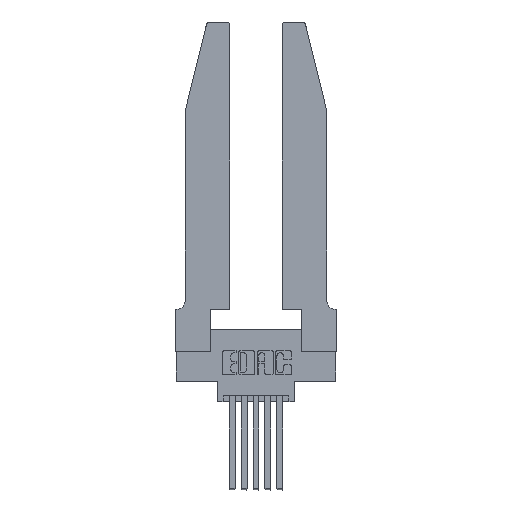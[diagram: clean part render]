
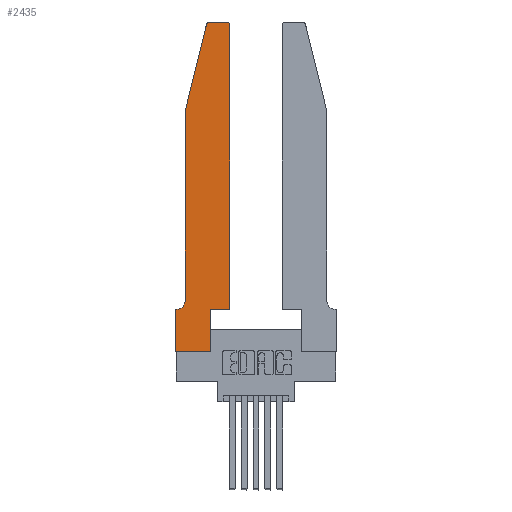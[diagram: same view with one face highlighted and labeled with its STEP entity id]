
A CAD part, top view. The second image highlights one B-rep face of the part: STEP entity #2435.
In plain terms, the highlighted planar face has unit normal (0, 0, 1).
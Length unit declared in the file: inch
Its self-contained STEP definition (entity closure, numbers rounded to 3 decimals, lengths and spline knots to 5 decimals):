
#417 = VERTEX_POINT ( 'NONE', #3624 ) ;
#426 = CARTESIAN_POINT ( 'NONE',  ( 0., 0., 0.37 ) ) ;
#519 = ORIENTED_EDGE ( 'NONE', *, *, #11851, .T. ) ;
#728 = VERTEX_POINT ( 'NONE', #12344 ) ;
#808 = EDGE_CURVE ( 'NONE', #11950, #12242, #9033, .T. ) ;
#812 = CARTESIAN_POINT ( 'NONE',  ( 0., 0., 0.37 ) ) ;
#825 = VECTOR ( 'NONE', #11538, 39.37008 ) ;
#841 = DIRECTION ( 'NONE',  ( 1., 0., 0. ) ) ;
#1068 = VERTEX_POINT ( 'NONE', #5139 ) ;
#1490 = CARTESIAN_POINT ( 'NONE',  ( 0.2605, 2.75, 0.37 ) ) ;
#1587 = ORIENTED_EDGE ( 'NONE', *, *, #10519, .T. ) ;
#1811 = DIRECTION ( 'NONE',  ( 0., -1., 0. ) ) ;
#1872 = VECTOR ( 'NONE', #1811, 39.37008 ) ;
#1958 = DIRECTION ( 'NONE',  ( 0., 0., -1. ) ) ;
#2183 = EDGE_CURVE ( 'NONE', #6797, #1068, #3558, .T. ) ;
#2215 = DIRECTION ( 'NONE',  ( 1., 0., 0. ) ) ;
#2264 = EDGE_CURVE ( 'NONE', #12815, #11950, #6085, .T. ) ;
#2298 = ORIENTED_EDGE ( 'NONE', *, *, #5454, .T. ) ;
#2426 = CARTESIAN_POINT ( 'NONE',  ( 0.4505, 0.35, 0.37 ) ) ;
#2435 = ADVANCED_FACE ( 'NONE', ( #12034 ), #10306, .T. ) ;
#2455 = CIRCLE ( 'NONE', #12380, 0.03 ) ;
#2553 = CARTESIAN_POINT ( 'NONE',  ( 0.2865, 0.35, 0.37 ) ) ;
#2884 = DIRECTION ( 'NONE',  ( -1., 0., 0. ) ) ;
#2959 = LINE ( 'NONE', #3098, #5844 ) ;
#3089 = CARTESIAN_POINT ( 'NONE',  ( 0.4505, 2.72, 0.37 ) ) ;
#3098 = CARTESIAN_POINT ( 'NONE',  ( 0.0755, 0.35, 0.37 ) ) ;
#3274 = EDGE_CURVE ( 'NONE', #417, #6653, #2959, .T. ) ;
#3336 = CARTESIAN_POINT ( 'NONE',  ( 0.284, 2.75, 0.37 ) ) ;
#3456 = ORIENTED_EDGE ( 'NONE', *, *, #3274, .T. ) ;
#3558 = CIRCLE ( 'NONE', #11795, 0.03 ) ;
#3624 = CARTESIAN_POINT ( 'NONE',  ( 0.0055, 0.35, 0.37 ) ) ;
#3635 = CARTESIAN_POINT ( 'NONE',  ( 0.0755, 2., 0.37 ) ) ;
#3970 = ORIENTED_EDGE ( 'NONE', *, *, #4714, .T. ) ;
#4210 = DIRECTION ( 'NONE',  ( -0.239, -0.971, 0. ) ) ;
#4459 = DIRECTION ( 'NONE',  ( 0., -1., 0. ) ) ;
#4629 = VECTOR ( 'NONE', #7908, 39.37008 ) ;
#4654 = EDGE_CURVE ( 'NONE', #9669, #6226, #7743, .T. ) ;
#4713 = DIRECTION ( 'NONE',  ( 0., 0., 1. ) ) ;
#4714 = EDGE_CURVE ( 'NONE', #9128, #6797, #12514, .T. ) ;
#4790 = CARTESIAN_POINT ( 'NONE',  ( 0.4505, 0.35, 0.37 ) ) ;
#4834 = ORIENTED_EDGE ( 'NONE', *, *, #4654, .T. ) ;
#4961 = VECTOR ( 'NONE', #5698, 39.37008 ) ;
#4978 = VECTOR ( 'NONE', #4210, 39.37008 ) ;
#5139 = CARTESIAN_POINT ( 'NONE',  ( 0.25487, 2.72718, 0.37 ) ) ;
#5454 = EDGE_CURVE ( 'NONE', #6653, #12815, #10328, .T. ) ;
#5479 = CARTESIAN_POINT ( 'NONE',  ( 0.4205, 2.75, 0.37 ) ) ;
#5698 = DIRECTION ( 'NONE',  ( 0., 1., 0. ) ) ;
#5844 = VECTOR ( 'NONE', #2884, 39.37008 ) ;
#6085 = LINE ( 'NONE', #812, #8509 ) ;
#6226 = VERTEX_POINT ( 'NONE', #3089 ) ;
#6653 = VERTEX_POINT ( 'NONE', #11190 ) ;
#6797 = VERTEX_POINT ( 'NONE', #3336 ) ;
#7358 = LINE ( 'NONE', #9672, #9467 ) ;
#7596 = LINE ( 'NONE', #4790, #10367 ) ;
#7743 = LINE ( 'NONE', #2426, #4961 ) ;
#7908 = DIRECTION ( 'NONE',  ( -1., 0., 0. ) ) ;
#7952 = EDGE_CURVE ( 'NONE', #12277, #728, #7358, .T. ) ;
#8076 = DIRECTION ( 'NONE',  ( 0., 0., 1. ) ) ;
#8120 = CARTESIAN_POINT ( 'NONE',  ( 0.284, 2.72, 0.37 ) ) ;
#8343 = CARTESIAN_POINT ( 'NONE',  ( 0.0055, 0.42, 0.37 ) ) ;
#8395 = CIRCLE ( 'NONE', #10869, 0.07 ) ;
#8509 = VECTOR ( 'NONE', #841, 39.37008 ) ;
#9033 = LINE ( 'NONE', #11475, #825 ) ;
#9128 = VERTEX_POINT ( 'NONE', #5479 ) ;
#9390 = DIRECTION ( 'NONE',  ( -1., 0., 0. ) ) ;
#9467 = VECTOR ( 'NONE', #4459, 39.37008 ) ;
#9669 = VERTEX_POINT ( 'NONE', #10265 ) ;
#9672 = CARTESIAN_POINT ( 'NONE',  ( 0.0755, 2., 0.37 ) ) ;
#9724 = ORIENTED_EDGE ( 'NONE', *, *, #2183, .T. ) ;
#9992 = DIRECTION ( 'NONE',  ( 1., 0., 0. ) ) ;
#10177 = AXIS2_PLACEMENT_3D ( 'NONE', #12998, #10236, #10488 ) ;
#10236 = DIRECTION ( 'NONE',  ( 0., 0., 1. ) ) ;
#10265 = CARTESIAN_POINT ( 'NONE',  ( 0.4505, 0.35, 0.37 ) ) ;
#10306 = PLANE ( 'NONE',  #10177 ) ;
#10328 = LINE ( 'NONE', #13235, #1872 ) ;
#10367 = VECTOR ( 'NONE', #9992, 39.37008 ) ;
#10488 = DIRECTION ( 'NONE',  ( 1., 0., 0. ) ) ;
#10504 = CARTESIAN_POINT ( 'NONE',  ( 0.0755, 2., 0.37 ) ) ;
#10519 = EDGE_CURVE ( 'NONE', #6226, #9128, #2455, .T. ) ;
#10727 = ORIENTED_EDGE ( 'NONE', *, *, #2264, .T. ) ;
#10869 = AXIS2_PLACEMENT_3D ( 'NONE', #8343, #1958, #9390 ) ;
#10956 = CARTESIAN_POINT ( 'NONE',  ( 0.4205, 2.72, 0.37 ) ) ;
#11184 = EDGE_CURVE ( 'NONE', #12242, #9669, #7596, .T. ) ;
#11190 = CARTESIAN_POINT ( 'NONE',  ( 0., 0.35, 0.37 ) ) ;
#11343 = ORIENTED_EDGE ( 'NONE', *, *, #808, .T. ) ;
#11461 = EDGE_CURVE ( 'NONE', #1068, #12277, #12832, .T. ) ;
#11475 = CARTESIAN_POINT ( 'NONE',  ( 0.2865, 0.35, 0.37 ) ) ;
#11538 = DIRECTION ( 'NONE',  ( 0., 1., 0. ) ) ;
#11795 = AXIS2_PLACEMENT_3D ( 'NONE', #8120, #8076, #2215 ) ;
#11851 = EDGE_CURVE ( 'NONE', #728, #417, #8395, .T. ) ;
#11950 = VERTEX_POINT ( 'NONE', #12550 ) ;
#11960 = DIRECTION ( 'NONE',  ( 1., 0., 0. ) ) ;
#12034 = FACE_OUTER_BOUND ( 'NONE', #13510, .T. ) ;
#12242 = VERTEX_POINT ( 'NONE', #2553 ) ;
#12277 = VERTEX_POINT ( 'NONE', #3635 ) ;
#12344 = CARTESIAN_POINT ( 'NONE',  ( 0.0755, 0.42, 0.37 ) ) ;
#12380 = AXIS2_PLACEMENT_3D ( 'NONE', #10956, #4713, #11960 ) ;
#12514 = LINE ( 'NONE', #1490, #4629 ) ;
#12550 = CARTESIAN_POINT ( 'NONE',  ( 0.2865, 0., 0.37 ) ) ;
#12815 = VERTEX_POINT ( 'NONE', #426 ) ;
#12832 = LINE ( 'NONE', #10504, #4978 ) ;
#12998 = CARTESIAN_POINT ( 'NONE',  ( 0., 0.35, 0.37 ) ) ;
#13010 = ORIENTED_EDGE ( 'NONE', *, *, #11461, .T. ) ;
#13235 = CARTESIAN_POINT ( 'NONE',  ( 0., 0., 0.37 ) ) ;
#13463 = ORIENTED_EDGE ( 'NONE', *, *, #7952, .T. ) ;
#13483 = ORIENTED_EDGE ( 'NONE', *, *, #11184, .T. ) ;
#13510 = EDGE_LOOP ( 'NONE', ( #3970, #9724, #13010, #13463, #519, #3456, #2298, #10727, #11343, #13483, #4834, #1587 ) ) ;
